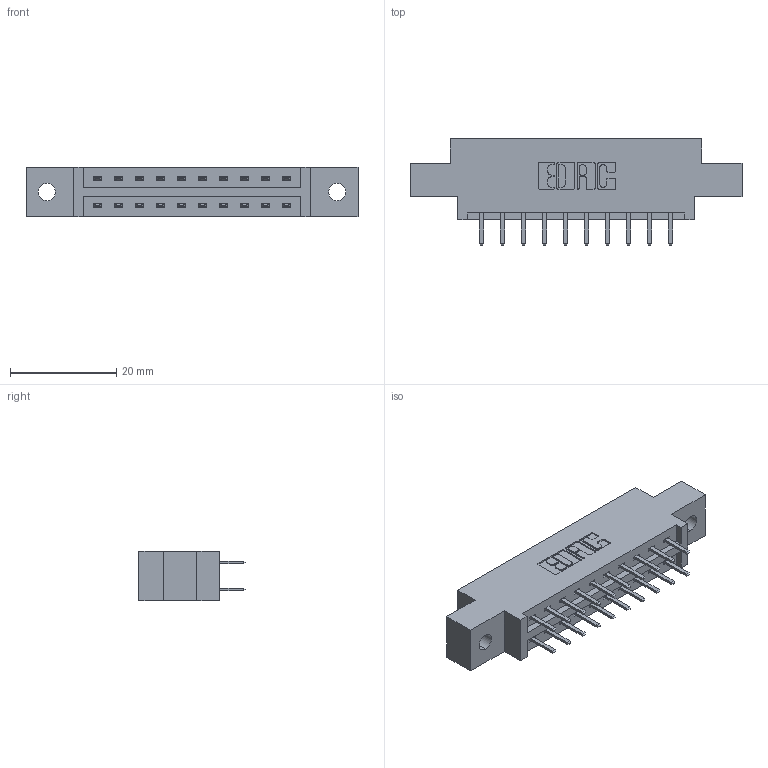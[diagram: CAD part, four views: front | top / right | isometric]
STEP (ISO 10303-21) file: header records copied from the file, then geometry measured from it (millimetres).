
FILE_DESCRIPTION (( 'STEP AP203' ), '1' );
FILE_NAME ('387-020-520-802.STEP', '2018-09-13T06:55:24', ( '' ), ( '' ), 'SwSTEP 2.0', 'SolidWorks 2016', '' );
FILE_SCHEMA (( 'CONFIG_CONTROL_DESIGN' ));
Length unit declared in the file: inch
Products named in the file (3): 337 Part_0.170 Offset - 0.128 Dia; 345-292-001_345-293-120; 387-020-520-802
Assembly tree (21 placements, depth 2):
  387-020-520-802
    337 Part_0.170 Offset - 0.128 Dia
    345-292-001_345-293-120  x20
Bounding box: 62.64 x 20.02 x 9.4 mm (x, y, z)
Volume: 6012.2 mm3; surface area: 6296 mm2
Topology: 21 solids, 21 shells, 1278 faces, 3703 edges, 2414 vertices
Faces by surface type: plane 874, cylinder 404
Entity records: 12141 total; most frequent: CARTESIAN_POINT 2086, ORIENTED_EDGE 2010, DIRECTION 1821, EDGE_CURVE 1005, LINE 873, VECTOR 873, VERTEX_POINT 666, AXIS2_PLACEMENT_3D 474
